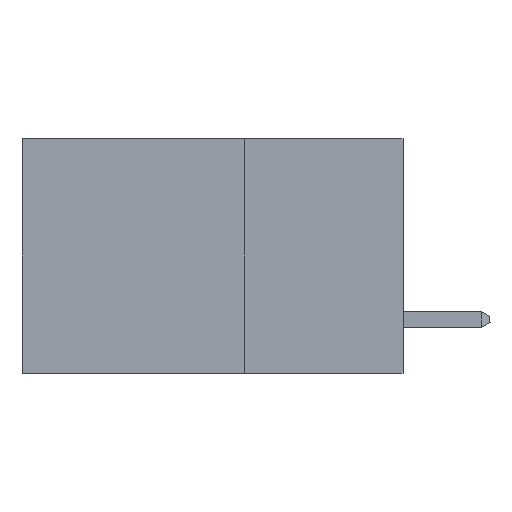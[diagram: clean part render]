
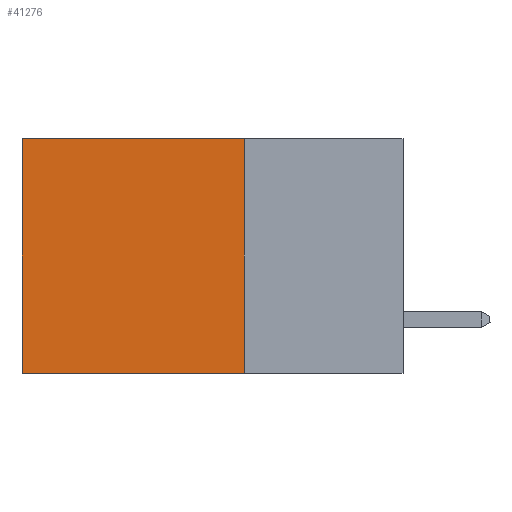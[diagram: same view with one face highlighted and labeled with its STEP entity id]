
A CAD part, left-side view. The second image highlights one B-rep face of the part: STEP entity #41276.
In plain terms, the highlighted planar face has unit normal (-1, 0, 0).
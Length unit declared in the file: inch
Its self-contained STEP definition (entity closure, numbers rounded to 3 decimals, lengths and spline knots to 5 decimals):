
#2332 = DIRECTION ( 'NONE',  ( 0., 0., -1. ) ) ;
#6186 = FACE_OUTER_BOUND ( 'NONE', #10647, .T. ) ;
#9138 = EDGE_CURVE ( 'NONE', #27639, #43582, #31811, .T. ) ;
#9350 = VERTEX_POINT ( 'NONE', #15309 ) ;
#10116 = DIRECTION ( 'NONE',  ( 0., 1., 0. ) ) ;
#10647 = EDGE_LOOP ( 'NONE', ( #28994, #44854, #24834, #46855 ) ) ;
#10654 = CARTESIAN_POINT ( 'NONE',  ( 0.2875, 0.25, 0. ) ) ;
#12896 = PLANE ( 'NONE',  #45923 ) ;
#15309 = CARTESIAN_POINT ( 'NONE',  ( 0.2875, 0.25, -0.37 ) ) ;
#16215 = CARTESIAN_POINT ( 'NONE',  ( 0.2875, 0.25, -0.37 ) ) ;
#16316 = CARTESIAN_POINT ( 'NONE',  ( 0.2875, 0.25, 0. ) ) ;
#16591 = CARTESIAN_POINT ( 'NONE',  ( 0.2875, 0.6, 0. ) ) ;
#16738 = CARTESIAN_POINT ( 'NONE',  ( 0.2875, 0.6, -0.37 ) ) ;
#17190 = DIRECTION ( 'NONE',  ( 0., 0., -1. ) ) ;
#21735 = VECTOR ( 'NONE', #33955, 39.37008 ) ;
#22130 = EDGE_CURVE ( 'NONE', #43582, #44294, #48346, .T. ) ;
#24834 = ORIENTED_EDGE ( 'NONE', *, *, #33471, .F. ) ;
#26498 = VECTOR ( 'NONE', #2332, 39.37008 ) ;
#27639 = VERTEX_POINT ( 'NONE', #37225 ) ;
#27773 = DIRECTION ( 'NONE',  ( 1., 0., 0. ) ) ;
#28994 = ORIENTED_EDGE ( 'NONE', *, *, #22130, .T. ) ;
#31811 = LINE ( 'NONE', #46451, #39147 ) ;
#31953 = VECTOR ( 'NONE', #10116, 39.37008 ) ;
#33204 = LINE ( 'NONE', #10654, #26498 ) ;
#33259 = CARTESIAN_POINT ( 'NONE',  ( 0.2875, 0.6, 0. ) ) ;
#33471 = EDGE_CURVE ( 'NONE', #27639, #9350, #33204, .T. ) ;
#33955 = DIRECTION ( 'NONE',  ( 0., 0., -1. ) ) ;
#34483 = LINE ( 'NONE', #16215, #31953 ) ;
#37225 = CARTESIAN_POINT ( 'NONE',  ( 0.2875, 0.25, 0. ) ) ;
#39147 = VECTOR ( 'NONE', #47423, 39.37008 ) ;
#41276 = ADVANCED_FACE ( 'NONE', ( #6186 ), #12896, .F. ) ;
#43582 = VERTEX_POINT ( 'NONE', #16591 ) ;
#44294 = VERTEX_POINT ( 'NONE', #16738 ) ;
#44854 = ORIENTED_EDGE ( 'NONE', *, *, #44983, .F. ) ;
#44983 = EDGE_CURVE ( 'NONE', #9350, #44294, #34483, .T. ) ;
#45923 = AXIS2_PLACEMENT_3D ( 'NONE', #16316, #27773, #17190 ) ;
#46451 = CARTESIAN_POINT ( 'NONE',  ( 0.2875, 0.25, 0. ) ) ;
#46855 = ORIENTED_EDGE ( 'NONE', *, *, #9138, .T. ) ;
#47423 = DIRECTION ( 'NONE',  ( 0., 1., 0. ) ) ;
#48346 = LINE ( 'NONE', #33259, #21735 ) ;
